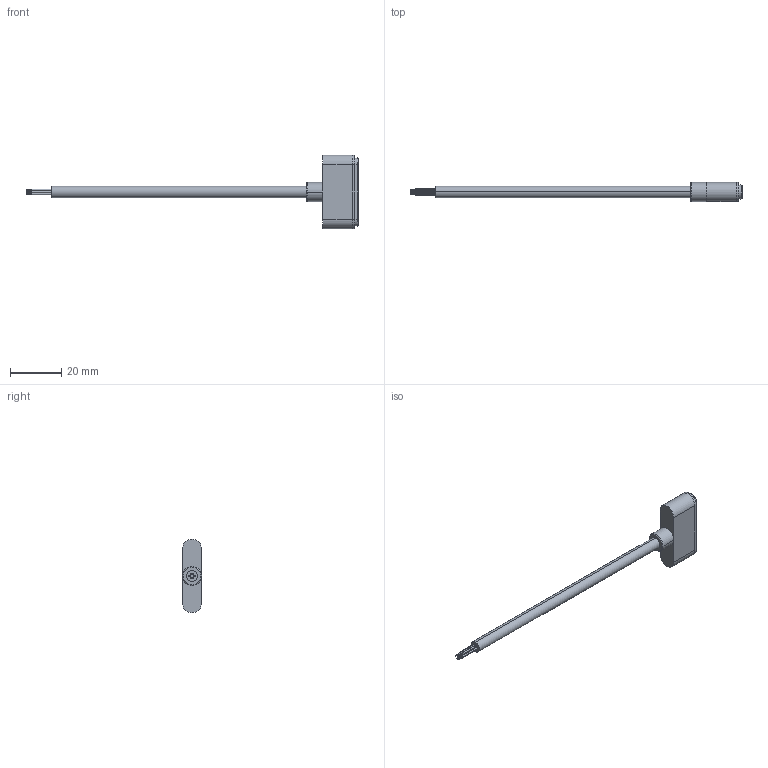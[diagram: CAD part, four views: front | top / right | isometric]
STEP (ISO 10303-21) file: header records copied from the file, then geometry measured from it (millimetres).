
FILE_DESCRIPTION (( 'STEP AP203' ), '1' );
FILE_NAME ('MCM-YA0-106-2R04VF10.STEP', '2025-11-25T16:04:41', ( '' ), ( '' ), 'SwSTEP 2.0', 'SolidWorks 2023', '' );
FILE_SCHEMA (( 'CONFIG_CONTROL_DESIGN' ));
Length unit declared in the file: millimetre
Products named in the file (1): MCM-YA0-106-2R04VF10
Bounding box: 130.15 x 7.5 x 28.9 mm (x, y, z)
Surface area: 3333.5 mm2 (no closed solid volume)
Topology: 0 solids, 15 shells, 147 faces, 382 edges, 250 vertices
Faces by surface type: cylinder 68, plane 39, torus 21, sphere 12, cone 5, bspline 2
Entity records: 4450 total; most frequent: DIRECTION 855, CARTESIAN_POINT 796, ORIENTED_EDGE 622, EDGE_CURVE 358, AXIS2_PLACEMENT_3D 357, VERTEX_POINT 238, CIRCLE 211, EDGE_LOOP 172
